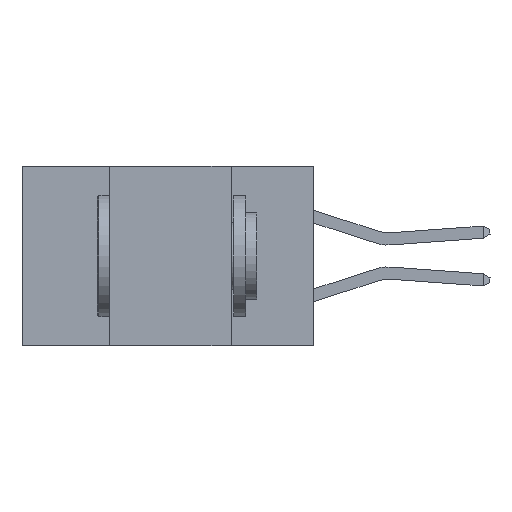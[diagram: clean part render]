
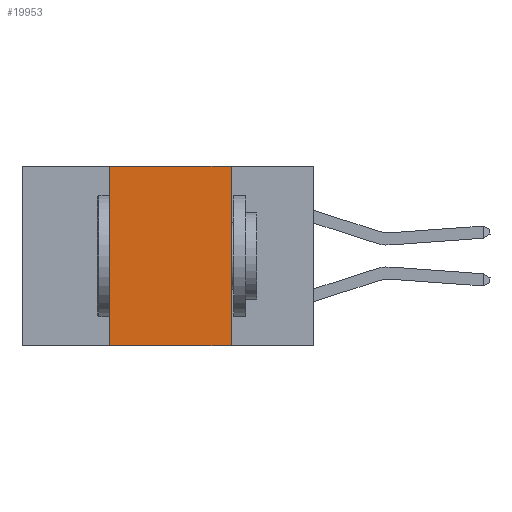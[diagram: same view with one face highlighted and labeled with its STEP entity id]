
A CAD part, left-side view. The second image highlights one B-rep face of the part: STEP entity #19953.
In plain terms, the highlighted planar face has unit normal (-1, 0, 0).
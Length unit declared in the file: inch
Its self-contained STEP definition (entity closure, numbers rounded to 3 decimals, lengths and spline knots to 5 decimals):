
#752 = CARTESIAN_POINT ( 'NONE',  ( 0., 0.6, 0. ) ) ;
#933 = DIRECTION ( 'NONE',  ( 0., 0., -1. ) ) ;
#2580 = VECTOR ( 'NONE', #10317, 39.37008 ) ;
#2796 = ORIENTED_EDGE ( 'NONE', *, *, #15427, .F. ) ;
#3127 = ORIENTED_EDGE ( 'NONE', *, *, #15227, .T. ) ;
#3689 = ORIENTED_EDGE ( 'NONE', *, *, #7506, .F. ) ;
#4857 = VECTOR ( 'NONE', #14886, 39.37008 ) ;
#5389 = DIRECTION ( 'NONE',  ( 1., 0., 0. ) ) ;
#5921 = FACE_OUTER_BOUND ( 'NONE', #10375, .T. ) ;
#6823 = CARTESIAN_POINT ( 'NONE',  ( 0., 0.42, -0.37 ) ) ;
#6947 = VERTEX_POINT ( 'NONE', #22508 ) ;
#7506 = EDGE_CURVE ( 'NONE', #9289, #9014, #8986, .T. ) ;
#7885 = CARTESIAN_POINT ( 'NONE',  ( 0., 0.17, 0. ) ) ;
#8466 = LINE ( 'NONE', #12823, #2580 ) ;
#8986 = LINE ( 'NONE', #25722, #4857 ) ;
#9014 = VERTEX_POINT ( 'NONE', #12827 ) ;
#9289 = VERTEX_POINT ( 'NONE', #6823 ) ;
#9552 = PLANE ( 'NONE',  #17823 ) ;
#10317 = DIRECTION ( 'NONE',  ( 0., -1., 0. ) ) ;
#10375 = EDGE_LOOP ( 'NONE', ( #25261, #2796, #3689, #3127 ) ) ;
#12823 = CARTESIAN_POINT ( 'NONE',  ( 0., 0.6, 0. ) ) ;
#12827 = CARTESIAN_POINT ( 'NONE',  ( 0., 0.42, 0. ) ) ;
#13943 = EDGE_CURVE ( 'NONE', #6947, #18273, #21652, .T. ) ;
#14562 = DIRECTION ( 'NONE',  ( 0., -1., 0. ) ) ;
#14703 = LINE ( 'NONE', #18871, #21572 ) ;
#14886 = DIRECTION ( 'NONE',  ( 0., 0., 1. ) ) ;
#15227 = EDGE_CURVE ( 'NONE', #9289, #18273, #14703, .T. ) ;
#15427 = EDGE_CURVE ( 'NONE', #9014, #6947, #8466, .T. ) ;
#17532 = VECTOR ( 'NONE', #21366, 39.37008 ) ;
#17823 = AXIS2_PLACEMENT_3D ( 'NONE', #752, #5389, #933 ) ;
#17891 = CARTESIAN_POINT ( 'NONE',  ( 0., 0.17, -0.37 ) ) ;
#18273 = VERTEX_POINT ( 'NONE', #17891 ) ;
#18871 = CARTESIAN_POINT ( 'NONE',  ( 0., 0.6, -0.37 ) ) ;
#19953 = ADVANCED_FACE ( 'NONE', ( #5921 ), #9552, .F. ) ;
#21366 = DIRECTION ( 'NONE',  ( 0., 0., -1. ) ) ;
#21572 = VECTOR ( 'NONE', #14562, 39.37008 ) ;
#21652 = LINE ( 'NONE', #7885, #17532 ) ;
#22508 = CARTESIAN_POINT ( 'NONE',  ( 0., 0.17, 0. ) ) ;
#25261 = ORIENTED_EDGE ( 'NONE', *, *, #13943, .F. ) ;
#25722 = CARTESIAN_POINT ( 'NONE',  ( 0., 0.42, 0. ) ) ;
